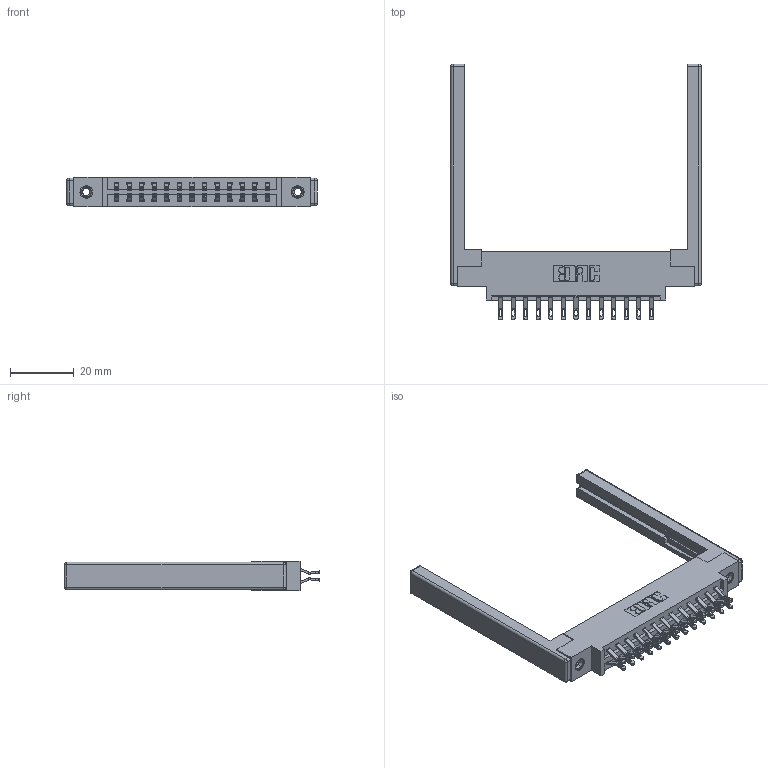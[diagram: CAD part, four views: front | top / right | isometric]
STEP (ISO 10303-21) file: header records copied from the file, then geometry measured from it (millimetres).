
FILE_DESCRIPTION (( 'STEP AP203' ), '1' );
FILE_NAME ('387-026-555-868.STEP', '2019-10-16T20:39:01', ( '' ), ( '' ), 'SwSTEP 2.0', 'SolidWorks 2016', '' );
FILE_SCHEMA (( 'CONFIG_CONTROL_DESIGN' ));
Length unit declared in the file: inch
Products named in the file (5): 345-250-001_345-250-001-102; 307-220-068; 345-292-001_555 Tail; 337 Part_0.170 Offset - 0.156 Dia-TI; 387-026-555-868
Assembly tree (31 placements, depth 2):
  387-026-555-868
    337 Part_0.170 Offset - 0.156 Dia-TI
    345-292-001_555 Tail  x26
    345-250-001_345-250-001-102  x2
    307-220-068  x2
Bounding box: 78.94 x 80.52 x 9.4 mm (x, y, z)
Volume: 12276.3 mm3; surface area: 13066.1 mm2
Topology: 31 solids, 31 shells, 1832 faces, 5627 edges, 3730 vertices
Faces by surface type: plane 1098, cylinder 710, cone 12, sphere 8, torus 4
Entity records: 17048 total; most frequent: CARTESIAN_POINT 2897, ORIENTED_EDGE 2792, DIRECTION 2558, EDGE_CURVE 1396, VECTOR 1198, LINE 1198, VERTEX_POINT 922, AXIS2_PLACEMENT_3D 680
